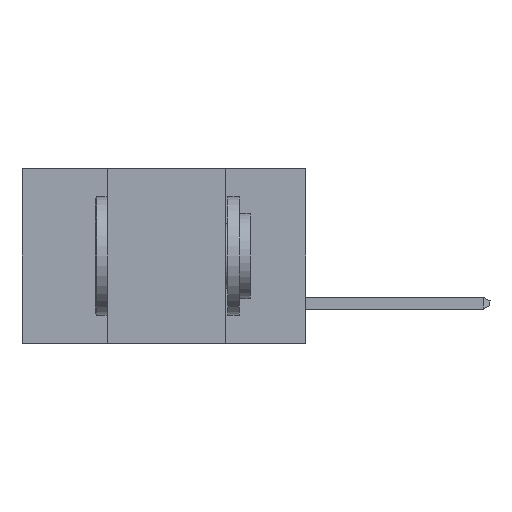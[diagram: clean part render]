
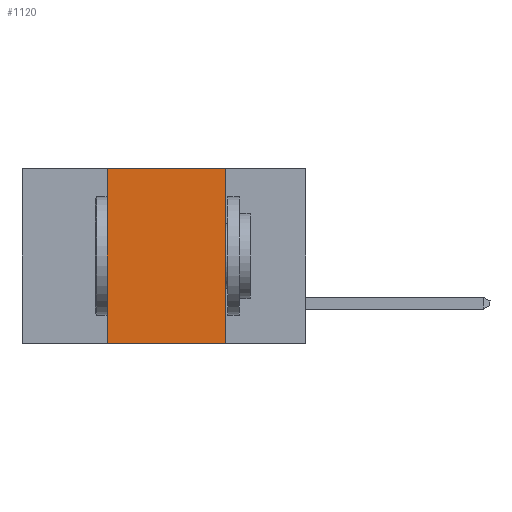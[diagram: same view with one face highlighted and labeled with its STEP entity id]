
A CAD part, left-side view. The second image highlights one B-rep face of the part: STEP entity #1120.
In plain terms, the highlighted planar face has unit normal (-1, 0, 0).
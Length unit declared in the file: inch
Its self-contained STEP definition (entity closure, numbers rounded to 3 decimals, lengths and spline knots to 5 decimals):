
#52 = VERTEX_POINT ( 'NONE', #10712 ) ;
#649 = DIRECTION ( 'NONE',  ( 1., 0., 0. ) ) ;
#971 = VERTEX_POINT ( 'NONE', #1387 ) ;
#1120 = ADVANCED_FACE ( 'NONE', ( #10016 ), #2544, .F. ) ;
#1387 = CARTESIAN_POINT ( 'NONE',  ( 0., 0.17, -0.37 ) ) ;
#1684 = DIRECTION ( 'NONE',  ( 0., -1., 0. ) ) ;
#2269 = LINE ( 'NONE', #7412, #8734 ) ;
#2517 = LINE ( 'NONE', #13045, #13194 ) ;
#2544 = PLANE ( 'NONE',  #10832 ) ;
#2933 = VECTOR ( 'NONE', #1684, 39.37008 ) ;
#2982 = EDGE_CURVE ( 'NONE', #52, #971, #2269, .T. ) ;
#3076 = EDGE_LOOP ( 'NONE', ( #5240, #11916, #9877, #9556 ) ) ;
#3956 = CARTESIAN_POINT ( 'NONE',  ( 0., 0.6, 0. ) ) ;
#4906 = LINE ( 'NONE', #3956, #2933 ) ;
#5240 = ORIENTED_EDGE ( 'NONE', *, *, #10038, .F. ) ;
#5654 = LINE ( 'NONE', #9830, #6287 ) ;
#6287 = VECTOR ( 'NONE', #11876, 39.37008 ) ;
#6499 = CARTESIAN_POINT ( 'NONE',  ( 0., 0.42, 0. ) ) ;
#7340 = EDGE_CURVE ( 'NONE', #52, #9888, #5654, .T. ) ;
#7412 = CARTESIAN_POINT ( 'NONE',  ( 0., 0.6, -0.37 ) ) ;
#8430 = VERTEX_POINT ( 'NONE', #12180 ) ;
#8734 = VECTOR ( 'NONE', #10676, 39.37008 ) ;
#8987 = DIRECTION ( 'NONE',  ( 0., 0., -1. ) ) ;
#9556 = ORIENTED_EDGE ( 'NONE', *, *, #2982, .T. ) ;
#9830 = CARTESIAN_POINT ( 'NONE',  ( 0., 0.42, -0.37 ) ) ;
#9877 = ORIENTED_EDGE ( 'NONE', *, *, #7340, .F. ) ;
#9888 = VERTEX_POINT ( 'NONE', #6499 ) ;
#10016 = FACE_OUTER_BOUND ( 'NONE', #3076, .T. ) ;
#10038 = EDGE_CURVE ( 'NONE', #8430, #971, #2517, .T. ) ;
#10676 = DIRECTION ( 'NONE',  ( 0., -1., 0. ) ) ;
#10712 = CARTESIAN_POINT ( 'NONE',  ( 0., 0.42, -0.37 ) ) ;
#10832 = AXIS2_PLACEMENT_3D ( 'NONE', #10956, #649, #8987 ) ;
#10956 = CARTESIAN_POINT ( 'NONE',  ( 0., 0.6, 0. ) ) ;
#11278 = EDGE_CURVE ( 'NONE', #9888, #8430, #4906, .T. ) ;
#11876 = DIRECTION ( 'NONE',  ( 0., 0., 1. ) ) ;
#11916 = ORIENTED_EDGE ( 'NONE', *, *, #11278, .F. ) ;
#12180 = CARTESIAN_POINT ( 'NONE',  ( 0., 0.17, 0. ) ) ;
#12844 = DIRECTION ( 'NONE',  ( 0., 0., -1. ) ) ;
#13045 = CARTESIAN_POINT ( 'NONE',  ( 0., 0.17, -0.37 ) ) ;
#13194 = VECTOR ( 'NONE', #12844, 39.37008 ) ;
